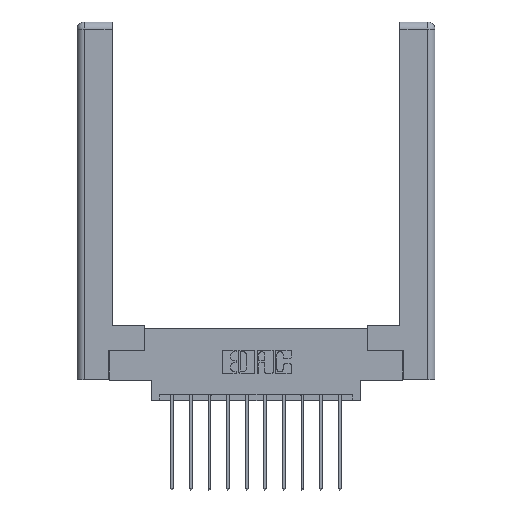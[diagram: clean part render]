
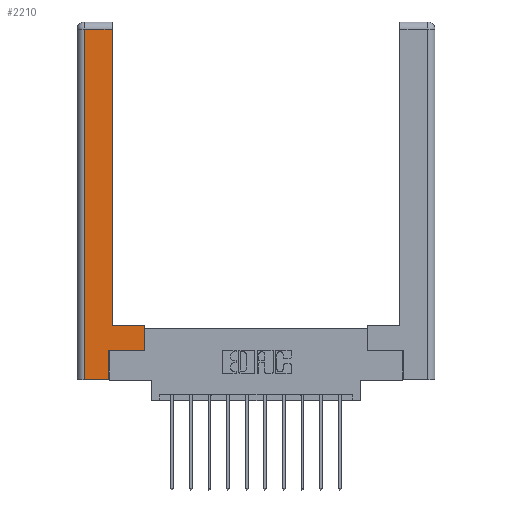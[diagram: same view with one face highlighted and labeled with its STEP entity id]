
A CAD part, top view. The second image highlights one B-rep face of the part: STEP entity #2210.
In plain terms, the highlighted planar face has unit normal (0, 0, 1).
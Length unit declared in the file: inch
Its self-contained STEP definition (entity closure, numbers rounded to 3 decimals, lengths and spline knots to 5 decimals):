
#319 = DIRECTION ( 'NONE',  ( 0., 1., 0. ) ) ;
#468 = CARTESIAN_POINT ( 'NONE',  ( 0.265, 0.245, 0. ) ) ;
#725 = EDGE_CURVE ( 'NONE', #7923, #10333, #8171, .T. ) ;
#735 = CARTESIAN_POINT ( 'NONE',  ( 0.0615, 2.94, 0. ) ) ;
#849 = LINE ( 'NONE', #12103, #3691 ) ;
#874 = DIRECTION ( 'NONE',  ( -1., 0., 0. ) ) ;
#1380 = CARTESIAN_POINT ( 'NONE',  ( 0.295, 0.45, 0. ) ) ;
#1666 = VECTOR ( 'NONE', #10217, 39.37008 ) ;
#1770 = VERTEX_POINT ( 'NONE', #13667 ) ;
#1915 = ORIENTED_EDGE ( 'NONE', *, *, #12436, .T. ) ;
#2210 = ADVANCED_FACE ( 'NONE', ( #3087 ), #9913, .F. ) ;
#2728 = VERTEX_POINT ( 'NONE', #5203 ) ;
#3087 = FACE_OUTER_BOUND ( 'NONE', #3099, .T. ) ;
#3099 = EDGE_LOOP ( 'NONE', ( #14175, #3813, #14214, #1915, #7339, #10782, #7328, #3759 ) ) ;
#3122 = EDGE_CURVE ( 'NONE', #10897, #2728, #14453, .T. ) ;
#3433 = CARTESIAN_POINT ( 'NONE',  ( 0.295, 3., 0. ) ) ;
#3682 = DIRECTION ( 'NONE',  ( 1., 0., 0. ) ) ;
#3691 = VECTOR ( 'NONE', #12244, 39.37008 ) ;
#3759 = ORIENTED_EDGE ( 'NONE', *, *, #8167, .T. ) ;
#3813 = ORIENTED_EDGE ( 'NONE', *, *, #725, .T. ) ;
#4058 = LINE ( 'NONE', #4425, #8874 ) ;
#4425 = CARTESIAN_POINT ( 'NONE',  ( 0.265, 0., 0. ) ) ;
#4550 = VERTEX_POINT ( 'NONE', #10744 ) ;
#4671 = LINE ( 'NONE', #10170, #1666 ) ;
#5068 = VECTOR ( 'NONE', #6782, 39.37008 ) ;
#5143 = CARTESIAN_POINT ( 'NONE',  ( 0.265, 0.245, 0. ) ) ;
#5157 = CARTESIAN_POINT ( 'NONE',  ( 0.0615, 0., 0. ) ) ;
#5203 = CARTESIAN_POINT ( 'NONE',  ( 0.565, 0.245, 0. ) ) ;
#5210 = VECTOR ( 'NONE', #319, 39.37008 ) ;
#6578 = VECTOR ( 'NONE', #12528, 39.37008 ) ;
#6782 = DIRECTION ( 'NONE',  ( -1., 0., 0. ) ) ;
#6855 = LINE ( 'NONE', #14668, #5068 ) ;
#7328 = ORIENTED_EDGE ( 'NONE', *, *, #13239, .T. ) ;
#7339 = ORIENTED_EDGE ( 'NONE', *, *, #8849, .T. ) ;
#7352 = LINE ( 'NONE', #468, #5210 ) ;
#7923 = VERTEX_POINT ( 'NONE', #11355 ) ;
#8167 = EDGE_CURVE ( 'NONE', #1770, #11264, #6855, .T. ) ;
#8171 = LINE ( 'NONE', #735, #13527 ) ;
#8765 = DIRECTION ( 'NONE',  ( 0., 0., -1. ) ) ;
#8849 = EDGE_CURVE ( 'NONE', #4550, #10897, #7352, .T. ) ;
#8874 = VECTOR ( 'NONE', #3682, 39.37008 ) ;
#9103 = CARTESIAN_POINT ( 'NONE',  ( 0.565, 0.245, 0. ) ) ;
#9534 = EDGE_CURVE ( 'NONE', #10333, #11575, #4671, .T. ) ;
#9648 = VECTOR ( 'NONE', #12717, 39.37008 ) ;
#9913 = PLANE ( 'NONE',  #11471 ) ;
#9960 = DIRECTION ( 'NONE',  ( -1., 0., 0. ) ) ;
#10170 = CARTESIAN_POINT ( 'NONE',  ( 0.0615, 0., 0. ) ) ;
#10217 = DIRECTION ( 'NONE',  ( 0., -1., 0. ) ) ;
#10333 = VERTEX_POINT ( 'NONE', #12348 ) ;
#10744 = CARTESIAN_POINT ( 'NONE',  ( 0.265, 0., 0. ) ) ;
#10782 = ORIENTED_EDGE ( 'NONE', *, *, #3122, .T. ) ;
#10897 = VERTEX_POINT ( 'NONE', #5143 ) ;
#11264 = VERTEX_POINT ( 'NONE', #1380 ) ;
#11273 = CARTESIAN_POINT ( 'NONE',  ( 0., 0., 0. ) ) ;
#11355 = CARTESIAN_POINT ( 'NONE',  ( 0.295, 2.94, 0. ) ) ;
#11471 = AXIS2_PLACEMENT_3D ( 'NONE', #11273, #8765, #9960 ) ;
#11575 = VERTEX_POINT ( 'NONE', #5157 ) ;
#12103 = CARTESIAN_POINT ( 'NONE',  ( 0.565, 0.45, 0. ) ) ;
#12244 = DIRECTION ( 'NONE',  ( 0., 1., 0. ) ) ;
#12348 = CARTESIAN_POINT ( 'NONE',  ( 0.0615, 2.94, 0. ) ) ;
#12366 = EDGE_CURVE ( 'NONE', #11264, #7923, #12673, .T. ) ;
#12436 = EDGE_CURVE ( 'NONE', #11575, #4550, #4058, .T. ) ;
#12528 = DIRECTION ( 'NONE',  ( 0., 1., 0. ) ) ;
#12673 = LINE ( 'NONE', #3433, #6578 ) ;
#12717 = DIRECTION ( 'NONE',  ( 1., 0., 0. ) ) ;
#13239 = EDGE_CURVE ( 'NONE', #2728, #1770, #849, .T. ) ;
#13527 = VECTOR ( 'NONE', #874, 39.37008 ) ;
#13667 = CARTESIAN_POINT ( 'NONE',  ( 0.565, 0.45, 0. ) ) ;
#14175 = ORIENTED_EDGE ( 'NONE', *, *, #12366, .T. ) ;
#14214 = ORIENTED_EDGE ( 'NONE', *, *, #9534, .T. ) ;
#14453 = LINE ( 'NONE', #9103, #9648 ) ;
#14668 = CARTESIAN_POINT ( 'NONE',  ( 0.295, 0.45, 0. ) ) ;
